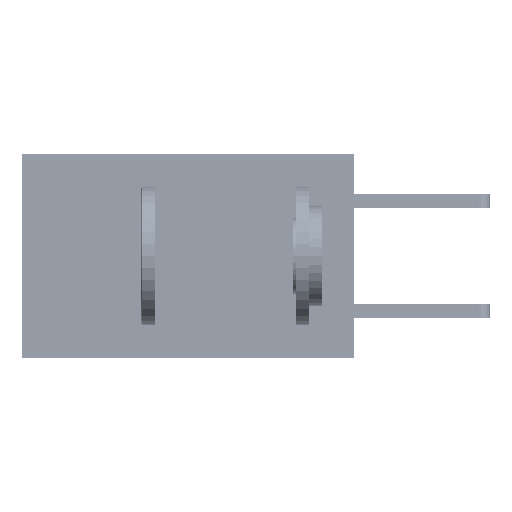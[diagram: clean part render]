
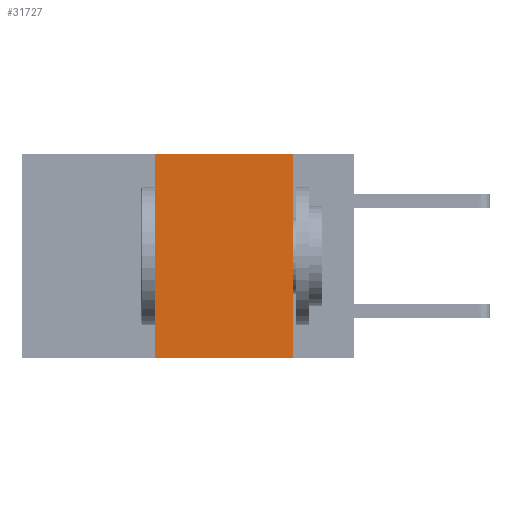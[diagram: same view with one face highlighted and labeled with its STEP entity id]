
A CAD part, left-side view. The second image highlights one B-rep face of the part: STEP entity #31727.
In plain terms, the highlighted planar face has unit normal (-1, 0, 0).
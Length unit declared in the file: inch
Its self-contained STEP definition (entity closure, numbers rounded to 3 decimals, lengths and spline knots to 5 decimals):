
#1167 = VECTOR ( 'NONE', #9502, 39.37008 ) ;
#1359 = VECTOR ( 'NONE', #1490, 39.37008 ) ;
#1490 = DIRECTION ( 'NONE',  ( 0., 0., 1. ) ) ;
#2289 = CARTESIAN_POINT ( 'NONE',  ( 0., 0.36, -0.37 ) ) ;
#3995 = CARTESIAN_POINT ( 'NONE',  ( 0., 0.11, -0.37 ) ) ;
#6800 = CARTESIAN_POINT ( 'NONE',  ( 0., 0.11, 0. ) ) ;
#8084 = ORIENTED_EDGE ( 'NONE', *, *, #20705, .F. ) ;
#9240 = LINE ( 'NONE', #44422, #35344 ) ;
#9502 = DIRECTION ( 'NONE',  ( 0., -1., 0. ) ) ;
#9819 = CARTESIAN_POINT ( 'NONE',  ( 0., 0.6, 0. ) ) ;
#11404 = FACE_OUTER_BOUND ( 'NONE', #16928, .T. ) ;
#11888 = ORIENTED_EDGE ( 'NONE', *, *, #25621, .F. ) ;
#12937 = LINE ( 'NONE', #24133, #1359 ) ;
#13928 = EDGE_CURVE ( 'NONE', #24968, #18705, #12937, .T. ) ;
#14852 = AXIS2_PLACEMENT_3D ( 'NONE', #23199, #20144, #23852 ) ;
#16928 = EDGE_LOOP ( 'NONE', ( #8084, #11888, #39436, #29018 ) ) ;
#17860 = DIRECTION ( 'NONE',  ( 0., -1., 0. ) ) ;
#18705 = VERTEX_POINT ( 'NONE', #31162 ) ;
#20144 = DIRECTION ( 'NONE',  ( 1., 0., 0. ) ) ;
#20705 = EDGE_CURVE ( 'NONE', #30611, #26948, #29480, .T. ) ;
#21556 = DIRECTION ( 'NONE',  ( 0., 0., -1. ) ) ;
#23199 = CARTESIAN_POINT ( 'NONE',  ( 0., 0.6, 0. ) ) ;
#23852 = DIRECTION ( 'NONE',  ( 0., 0., -1. ) ) ;
#24133 = CARTESIAN_POINT ( 'NONE',  ( 0., 0.36, 0. ) ) ;
#24968 = VERTEX_POINT ( 'NONE', #2289 ) ;
#25621 = EDGE_CURVE ( 'NONE', #18705, #30611, #40011, .T. ) ;
#26948 = VERTEX_POINT ( 'NONE', #3995 ) ;
#29018 = ORIENTED_EDGE ( 'NONE', *, *, #41876, .T. ) ;
#29480 = LINE ( 'NONE', #6800, #34130 ) ;
#30376 = CARTESIAN_POINT ( 'NONE',  ( 0., 0.11, 0. ) ) ;
#30387 = PLANE ( 'NONE',  #14852 ) ;
#30611 = VERTEX_POINT ( 'NONE', #30376 ) ;
#31162 = CARTESIAN_POINT ( 'NONE',  ( 0., 0.36, 0. ) ) ;
#31727 = ADVANCED_FACE ( 'NONE', ( #11404 ), #30387, .F. ) ;
#34130 = VECTOR ( 'NONE', #21556, 39.37008 ) ;
#35344 = VECTOR ( 'NONE', #17860, 39.37008 ) ;
#39436 = ORIENTED_EDGE ( 'NONE', *, *, #13928, .F. ) ;
#40011 = LINE ( 'NONE', #9819, #1167 ) ;
#41876 = EDGE_CURVE ( 'NONE', #24968, #26948, #9240, .T. ) ;
#44422 = CARTESIAN_POINT ( 'NONE',  ( 0., 0.6, -0.37 ) ) ;
